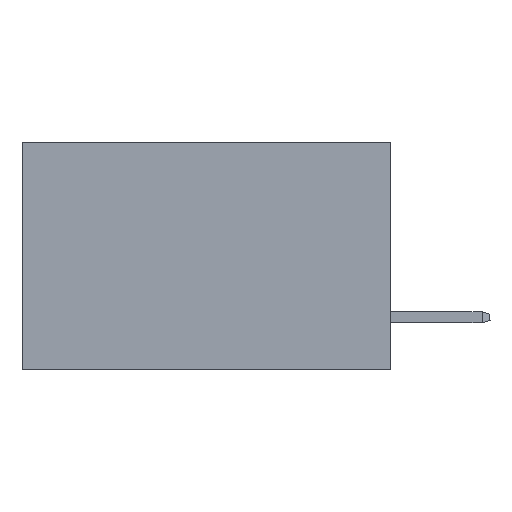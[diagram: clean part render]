
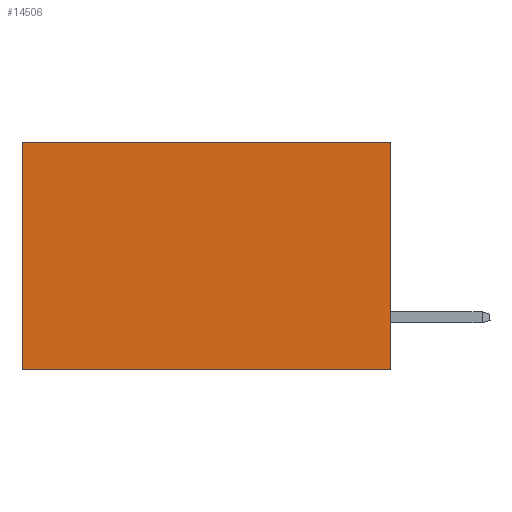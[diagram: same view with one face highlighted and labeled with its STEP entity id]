
A CAD part, left-side view. The second image highlights one B-rep face of the part: STEP entity #14506.
In plain terms, the highlighted planar face has unit normal (-1, 0, 0).
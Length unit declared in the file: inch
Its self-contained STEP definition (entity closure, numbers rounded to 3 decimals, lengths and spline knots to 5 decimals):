
#1784 = ORIENTED_EDGE ( 'NONE', *, *, #17951, .T. ) ;
#2071 = DIRECTION ( 'NONE',  ( 0., 0., -1. ) ) ;
#3506 = ORIENTED_EDGE ( 'NONE', *, *, #18609, .F. ) ;
#4697 = CARTESIAN_POINT ( 'NONE',  ( 0.2875, 0.6, -0.37 ) ) ;
#4812 = CARTESIAN_POINT ( 'NONE',  ( 0.2875, 0., -0.37 ) ) ;
#4845 = ORIENTED_EDGE ( 'NONE', *, *, #7967, .T. ) ;
#5210 = LINE ( 'NONE', #14227, #8182 ) ;
#5840 = CARTESIAN_POINT ( 'NONE',  ( 0.2875, 0., -0.37 ) ) ;
#5873 = VECTOR ( 'NONE', #7360, 39.37008 ) ;
#6055 = LINE ( 'NONE', #13094, #11361 ) ;
#6164 = DIRECTION ( 'NONE',  ( 0., 0., -1. ) ) ;
#6248 = PLANE ( 'NONE',  #8838 ) ;
#6618 = VERTEX_POINT ( 'NONE', #4697 ) ;
#6924 = DIRECTION ( 'NONE',  ( 0., 0., -1. ) ) ;
#7116 = VERTEX_POINT ( 'NONE', #4812 ) ;
#7360 = DIRECTION ( 'NONE',  ( 0., 1., 0. ) ) ;
#7707 = CARTESIAN_POINT ( 'NONE',  ( 0.2875, 0., 0. ) ) ;
#7865 = CARTESIAN_POINT ( 'NONE',  ( 0.2875, 0.6, 0. ) ) ;
#7967 = EDGE_CURVE ( 'NONE', #8680, #13127, #6055, .T. ) ;
#8182 = VECTOR ( 'NONE', #6924, 39.37008 ) ;
#8611 = CARTESIAN_POINT ( 'NONE',  ( 0.2875, 0., 0. ) ) ;
#8680 = VERTEX_POINT ( 'NONE', #8611 ) ;
#8838 = AXIS2_PLACEMENT_3D ( 'NONE', #7707, #18163, #2071 ) ;
#10269 = CARTESIAN_POINT ( 'NONE',  ( 0.2875, 0.6, 0. ) ) ;
#10681 = LINE ( 'NONE', #5840, #5873 ) ;
#11009 = EDGE_LOOP ( 'NONE', ( #1784, #3506, #15342, #4845 ) ) ;
#11361 = VECTOR ( 'NONE', #13214, 39.37008 ) ;
#13094 = CARTESIAN_POINT ( 'NONE',  ( 0.2875, 0., 0. ) ) ;
#13127 = VERTEX_POINT ( 'NONE', #7865 ) ;
#13214 = DIRECTION ( 'NONE',  ( 0., 1., 0. ) ) ;
#14227 = CARTESIAN_POINT ( 'NONE',  ( 0.2875, 0., 0. ) ) ;
#14506 = ADVANCED_FACE ( 'NONE', ( #16248 ), #6248, .F. ) ;
#15298 = EDGE_CURVE ( 'NONE', #8680, #7116, #5210, .T. ) ;
#15342 = ORIENTED_EDGE ( 'NONE', *, *, #15298, .F. ) ;
#16248 = FACE_OUTER_BOUND ( 'NONE', #11009, .T. ) ;
#16897 = LINE ( 'NONE', #10269, #17392 ) ;
#17392 = VECTOR ( 'NONE', #6164, 39.37008 ) ;
#17951 = EDGE_CURVE ( 'NONE', #13127, #6618, #16897, .T. ) ;
#18163 = DIRECTION ( 'NONE',  ( 1., 0., 0. ) ) ;
#18609 = EDGE_CURVE ( 'NONE', #7116, #6618, #10681, .T. ) ;
